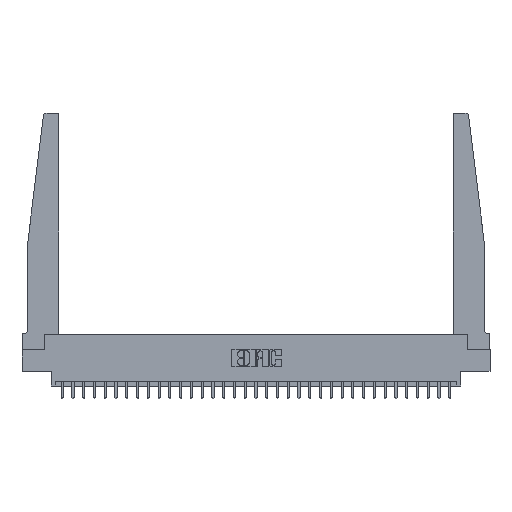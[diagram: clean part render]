
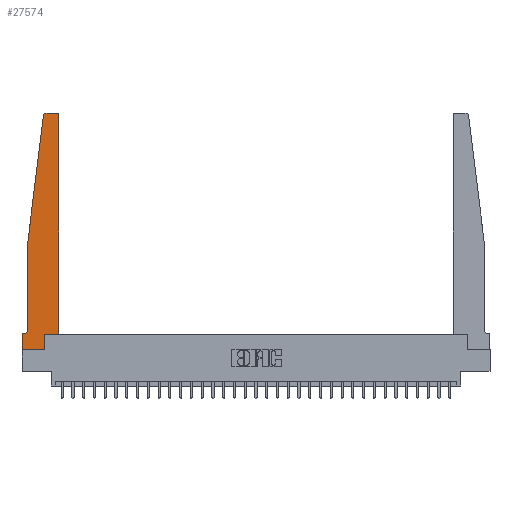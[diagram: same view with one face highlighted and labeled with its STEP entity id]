
A CAD part, top view. The second image highlights one B-rep face of the part: STEP entity #27574.
In plain terms, the highlighted planar face has unit normal (0, 0, 1).
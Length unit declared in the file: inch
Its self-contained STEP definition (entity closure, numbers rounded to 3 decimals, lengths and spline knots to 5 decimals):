
#722 = DIRECTION ( 'NONE',  ( 1., 0., 0. ) ) ;
#906 = CARTESIAN_POINT ( 'NONE',  ( 0.425, 2.72, 0.37 ) ) ;
#915 = PLANE ( 'NONE',  #8354 ) ;
#1014 = CARTESIAN_POINT ( 'NONE',  ( 0., 0.1875, 0.37 ) ) ;
#1140 = EDGE_LOOP ( 'NONE', ( #28486, #26209, #2314, #23300, #18607, #12354, #20562, #19426, #13212, #26652, #6004, #15220 ) ) ;
#2073 = CARTESIAN_POINT ( 'NONE',  ( 0.425, 0.18, 0.37 ) ) ;
#2314 = ORIENTED_EDGE ( 'NONE', *, *, #9240, .T. ) ;
#2411 = CARTESIAN_POINT ( 'NONE',  ( 0.395, 2.75, 0.37 ) ) ;
#3230 = CARTESIAN_POINT ( 'NONE',  ( 0.425, 0.18, 0.37 ) ) ;
#3329 = DIRECTION ( 'NONE',  ( 0., 0., 1. ) ) ;
#4211 = VECTOR ( 'NONE', #27059, 39.37008 ) ;
#4835 = LINE ( 'NONE', #24436, #22397 ) ;
#4882 = VECTOR ( 'NONE', #10483, 39.37008 ) ;
#5168 = FACE_OUTER_BOUND ( 'NONE', #1140, .T. ) ;
#5195 = CARTESIAN_POINT ( 'NONE',  ( 0.425, 0.18, 0.37 ) ) ;
#5470 = VECTOR ( 'NONE', #18006, 39.37008 ) ;
#5518 = DIRECTION ( 'NONE',  ( 1., 0., 0. ) ) ;
#5916 = EDGE_CURVE ( 'NONE', #20272, #28539, #11542, .T. ) ;
#6004 = ORIENTED_EDGE ( 'NONE', *, *, #28113, .T. ) ;
#6010 = EDGE_CURVE ( 'NONE', #28539, #22070, #14757, .T. ) ;
#6683 = VECTOR ( 'NONE', #16729, 39.37008 ) ;
#7061 = CIRCLE ( 'NONE', #13950, 0.03 ) ;
#7083 = CARTESIAN_POINT ( 'NONE',  ( 0.015, 0.1875, 0.37 ) ) ;
#7170 = CARTESIAN_POINT ( 'NONE',  ( 0.395, 2.72, 0.37 ) ) ;
#7182 = LINE ( 'NONE', #22737, #12551 ) ;
#7287 = CIRCLE ( 'NONE', #22823, 0.03 ) ;
#8354 = AXIS2_PLACEMENT_3D ( 'NONE', #1014, #3329, #19371 ) ;
#8416 = VECTOR ( 'NONE', #5518, 39.37008 ) ;
#8927 = CARTESIAN_POINT ( 'NONE',  ( 0.015, 0.2375, 0.37 ) ) ;
#9152 = VERTEX_POINT ( 'NONE', #15586 ) ;
#9162 = LINE ( 'NONE', #3230, #8416 ) ;
#9240 = EDGE_CURVE ( 'NONE', #11284, #14044, #7182, .T. ) ;
#9428 = CARTESIAN_POINT ( 'NONE',  ( 0.065, 1.25, 0.37 ) ) ;
#9485 = DIRECTION ( 'NONE',  ( 1., 0., 0. ) ) ;
#10483 = DIRECTION ( 'NONE',  ( -1., 0., 0. ) ) ;
#11240 = DIRECTION ( 'NONE',  ( -1., 0., 0. ) ) ;
#11284 = VERTEX_POINT ( 'NONE', #23376 ) ;
#11418 = DIRECTION ( 'NONE',  ( 0., -1., 0. ) ) ;
#11430 = VERTEX_POINT ( 'NONE', #906 ) ;
#11542 = LINE ( 'NONE', #24475, #5470 ) ;
#11708 = LINE ( 'NONE', #13280, #4211 ) ;
#11719 = EDGE_CURVE ( 'NONE', #14044, #24714, #11708, .T. ) ;
#12354 = ORIENTED_EDGE ( 'NONE', *, *, #5916, .T. ) ;
#12551 = VECTOR ( 'NONE', #15898, 39.37008 ) ;
#12672 = CARTESIAN_POINT ( 'NONE',  ( 0.065, 0.2375, 0.37 ) ) ;
#13212 = ORIENTED_EDGE ( 'NONE', *, *, #29476, .T. ) ;
#13280 = CARTESIAN_POINT ( 'NONE',  ( 0.065, 1.25, 0.37 ) ) ;
#13472 = LINE ( 'NONE', #5195, #6683 ) ;
#13950 = AXIS2_PLACEMENT_3D ( 'NONE', #7170, #23257, #9485 ) ;
#14044 = VERTEX_POINT ( 'NONE', #9428 ) ;
#14253 = EDGE_CURVE ( 'NONE', #22070, #27433, #17336, .T. ) ;
#14428 = DIRECTION ( 'NONE',  ( 0., 0., 1. ) ) ;
#14757 = LINE ( 'NONE', #25180, #28463 ) ;
#15220 = ORIENTED_EDGE ( 'NONE', *, *, #16503, .T. ) ;
#15586 = CARTESIAN_POINT ( 'NONE',  ( 0.2605, 0.18, 0.37 ) ) ;
#15898 = DIRECTION ( 'NONE',  ( -0.122, -0.992, 0. ) ) ;
#16451 = AXIS2_PLACEMENT_3D ( 'NONE', #8927, #25012, #11240 ) ;
#16503 = EDGE_CURVE ( 'NONE', #11430, #20227, #7061, .T. ) ;
#16729 = DIRECTION ( 'NONE',  ( 0., 1., 0. ) ) ;
#17336 = LINE ( 'NONE', #26192, #28833 ) ;
#17381 = EDGE_CURVE ( 'NONE', #9152, #18328, #9162, .T. ) ;
#17547 = EDGE_CURVE ( 'NONE', #20227, #20260, #29323, .T. ) ;
#18006 = DIRECTION ( 'NONE',  ( -1., 0., 0. ) ) ;
#18209 = CARTESIAN_POINT ( 'NONE',  ( 0., 0., 0.37 ) ) ;
#18328 = VERTEX_POINT ( 'NONE', #2073 ) ;
#18607 = ORIENTED_EDGE ( 'NONE', *, *, #25608, .T. ) ;
#19371 = DIRECTION ( 'NONE',  ( 1., 0., 0. ) ) ;
#19426 = ORIENTED_EDGE ( 'NONE', *, *, #14253, .T. ) ;
#20227 = VERTEX_POINT ( 'NONE', #2411 ) ;
#20260 = VERTEX_POINT ( 'NONE', #20768 ) ;
#20272 = VERTEX_POINT ( 'NONE', #7083 ) ;
#20562 = ORIENTED_EDGE ( 'NONE', *, *, #6010, .T. ) ;
#20768 = CARTESIAN_POINT ( 'NONE',  ( 0.27653, 2.75, 0.37 ) ) ;
#22070 = VERTEX_POINT ( 'NONE', #18209 ) ;
#22397 = VECTOR ( 'NONE', #26759, 39.37008 ) ;
#22438 = CIRCLE ( 'NONE', #16451, 0.05 ) ;
#22614 = CARTESIAN_POINT ( 'NONE',  ( 0., 0.1875, 0.37 ) ) ;
#22737 = CARTESIAN_POINT ( 'NONE',  ( 0.065, 1.25, 0.37 ) ) ;
#22823 = AXIS2_PLACEMENT_3D ( 'NONE', #28224, #14428, #722 ) ;
#23257 = DIRECTION ( 'NONE',  ( 0., 0., 1. ) ) ;
#23300 = ORIENTED_EDGE ( 'NONE', *, *, #11719, .T. ) ;
#23376 = CARTESIAN_POINT ( 'NONE',  ( 0.24675, 2.72367, 0.37 ) ) ;
#24436 = CARTESIAN_POINT ( 'NONE',  ( 0.2605, 0.18, 0.37 ) ) ;
#24475 = CARTESIAN_POINT ( 'NONE',  ( 0.065, 0.1875, 0.37 ) ) ;
#24714 = VERTEX_POINT ( 'NONE', #12672 ) ;
#25012 = DIRECTION ( 'NONE',  ( 0., 0., -1. ) ) ;
#25180 = CARTESIAN_POINT ( 'NONE',  ( 0., 0., 0.37 ) ) ;
#25608 = EDGE_CURVE ( 'NONE', #24714, #20272, #22438, .T. ) ;
#26192 = CARTESIAN_POINT ( 'NONE',  ( 0., 0., 0.37 ) ) ;
#26209 = ORIENTED_EDGE ( 'NONE', *, *, #27525, .T. ) ;
#26565 = CARTESIAN_POINT ( 'NONE',  ( 0.25, 2.75, 0.37 ) ) ;
#26652 = ORIENTED_EDGE ( 'NONE', *, *, #17381, .T. ) ;
#26759 = DIRECTION ( 'NONE',  ( 0., 1., 0. ) ) ;
#27059 = DIRECTION ( 'NONE',  ( 0., -1., 0. ) ) ;
#27433 = VERTEX_POINT ( 'NONE', #27627 ) ;
#27525 = EDGE_CURVE ( 'NONE', #20260, #11284, #7287, .T. ) ;
#27574 = ADVANCED_FACE ( 'NONE', ( #5168 ), #915, .T. ) ;
#27627 = CARTESIAN_POINT ( 'NONE',  ( 0.2605, 0., 0.37 ) ) ;
#28113 = EDGE_CURVE ( 'NONE', #18328, #11430, #13472, .T. ) ;
#28224 = CARTESIAN_POINT ( 'NONE',  ( 0.27653, 2.72, 0.37 ) ) ;
#28463 = VECTOR ( 'NONE', #11418, 39.37008 ) ;
#28486 = ORIENTED_EDGE ( 'NONE', *, *, #17547, .T. ) ;
#28530 = DIRECTION ( 'NONE',  ( 1., 0., 0. ) ) ;
#28539 = VERTEX_POINT ( 'NONE', #22614 ) ;
#28833 = VECTOR ( 'NONE', #28530, 39.37008 ) ;
#29323 = LINE ( 'NONE', #26565, #4882 ) ;
#29476 = EDGE_CURVE ( 'NONE', #27433, #9152, #4835, .T. ) ;
